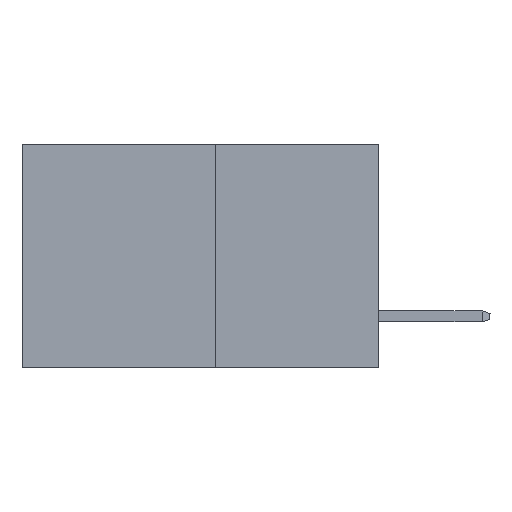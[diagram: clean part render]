
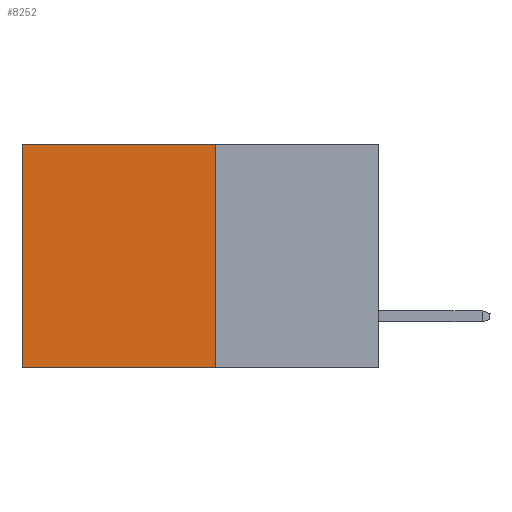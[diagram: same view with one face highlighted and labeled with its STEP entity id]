
A CAD part, left-side view. The second image highlights one B-rep face of the part: STEP entity #8252.
In plain terms, the highlighted planar face has unit normal (-1, 0, 0).
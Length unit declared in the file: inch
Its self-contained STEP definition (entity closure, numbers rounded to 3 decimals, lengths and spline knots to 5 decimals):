
#84 = CARTESIAN_POINT ( 'NONE',  ( 0.277, 0.27, -0.37 ) ) ;
#6235 = EDGE_CURVE ( 'NONE', #25753, #10600, #19116, .T. ) ;
#6938 = CARTESIAN_POINT ( 'NONE',  ( 0.277, 0.59, 0. ) ) ;
#7616 = EDGE_CURVE ( 'NONE', #10600, #23170, #20204, .T. ) ;
#8252 = ADVANCED_FACE ( 'NONE', ( #16203 ), #25471, .F. ) ;
#10600 = VERTEX_POINT ( 'NONE', #13357 ) ;
#10788 = CARTESIAN_POINT ( 'NONE',  ( 0.277, 0.59, -0.37 ) ) ;
#11901 = VECTOR ( 'NONE', #20634, 39.37008 ) ;
#12034 = CARTESIAN_POINT ( 'NONE',  ( 0.277, 0.27, 0. ) ) ;
#13357 = CARTESIAN_POINT ( 'NONE',  ( 0.277, 0.27, -0.37 ) ) ;
#13466 = VECTOR ( 'NONE', #23786, 39.37008 ) ;
#16203 = FACE_OUTER_BOUND ( 'NONE', #30678, .T. ) ;
#18310 = VECTOR ( 'NONE', #21199, 39.37008 ) ;
#19116 = LINE ( 'NONE', #21627, #18310 ) ;
#19541 = ORIENTED_EDGE ( 'NONE', *, *, #26729, .T. ) ;
#19895 = ORIENTED_EDGE ( 'NONE', *, *, #6235, .F. ) ;
#20204 = LINE ( 'NONE', #84, #13466 ) ;
#20288 = LINE ( 'NONE', #10788, #32853 ) ;
#20634 = DIRECTION ( 'NONE',  ( 0., 1., 0. ) ) ;
#21199 = DIRECTION ( 'NONE',  ( 0., 0., -1. ) ) ;
#21627 = CARTESIAN_POINT ( 'NONE',  ( 0.277, 0.27, -0.37 ) ) ;
#23170 = VERTEX_POINT ( 'NONE', #31067 ) ;
#23786 = DIRECTION ( 'NONE',  ( 0., 1., 0. ) ) ;
#25471 = PLANE ( 'NONE',  #27060 ) ;
#25584 = CARTESIAN_POINT ( 'NONE',  ( 0.277, 0.27, -0.37 ) ) ;
#25753 = VERTEX_POINT ( 'NONE', #12034 ) ;
#26042 = DIRECTION ( 'NONE',  ( 0., 0., -1. ) ) ;
#26240 = LINE ( 'NONE', #30653, #11901 ) ;
#26729 = EDGE_CURVE ( 'NONE', #25753, #27101, #26240, .T. ) ;
#27060 = AXIS2_PLACEMENT_3D ( 'NONE', #25584, #27668, #27560 ) ;
#27101 = VERTEX_POINT ( 'NONE', #6938 ) ;
#27560 = DIRECTION ( 'NONE',  ( 0., 0., -1. ) ) ;
#27668 = DIRECTION ( 'NONE',  ( 1., 0., 0. ) ) ;
#29485 = ORIENTED_EDGE ( 'NONE', *, *, #32298, .T. ) ;
#30615 = ORIENTED_EDGE ( 'NONE', *, *, #7616, .F. ) ;
#30653 = CARTESIAN_POINT ( 'NONE',  ( 0.277, 0.27, 0. ) ) ;
#30678 = EDGE_LOOP ( 'NONE', ( #29485, #30615, #19895, #19541 ) ) ;
#31067 = CARTESIAN_POINT ( 'NONE',  ( 0.277, 0.59, -0.37 ) ) ;
#32298 = EDGE_CURVE ( 'NONE', #27101, #23170, #20288, .T. ) ;
#32853 = VECTOR ( 'NONE', #26042, 39.37008 ) ;
